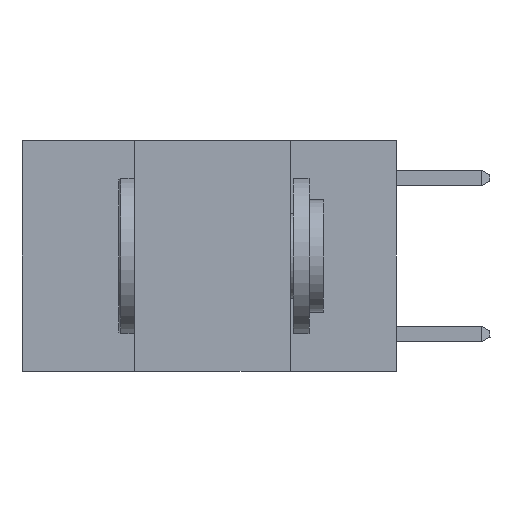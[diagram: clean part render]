
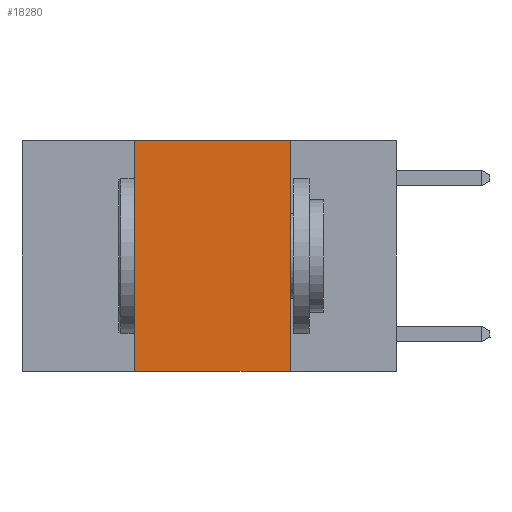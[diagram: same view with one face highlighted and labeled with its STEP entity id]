
A CAD part, left-side view. The second image highlights one B-rep face of the part: STEP entity #18280.
In plain terms, the highlighted planar face has unit normal (-1, 0, 0).
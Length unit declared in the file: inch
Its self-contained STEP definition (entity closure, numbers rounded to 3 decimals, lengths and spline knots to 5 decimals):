
#63 = VERTEX_POINT ( 'NONE', #12417 ) ;
#98 = CARTESIAN_POINT ( 'NONE',  ( 0., 0.42, -0.37 ) ) ;
#126 = CARTESIAN_POINT ( 'NONE',  ( 0., 0.6, 0. ) ) ;
#166 = LINE ( 'NONE', #17073, #260 ) ;
#260 = VECTOR ( 'NONE', #4436, 39.37008 ) ;
#839 = CARTESIAN_POINT ( 'NONE',  ( 0., 0.6, -0.37 ) ) ;
#1526 = EDGE_LOOP ( 'NONE', ( #18100, #18218, #18236, #18349 ) ) ;
#2316 = CARTESIAN_POINT ( 'NONE',  ( 0., 0.17, 0. ) ) ;
#2653 = CARTESIAN_POINT ( 'NONE',  ( 0., 0.42, 0. ) ) ;
#3962 = AXIS2_PLACEMENT_3D ( 'NONE', #126, #17803, #8577 ) ;
#4436 = DIRECTION ( 'NONE',  ( 0., -1., 0. ) ) ;
#5456 = VERTEX_POINT ( 'NONE', #18423 ) ;
#5472 = EDGE_CURVE ( 'NONE', #63, #5456, #166, .T. ) ;
#5507 = LINE ( 'NONE', #839, #5608 ) ;
#5608 = VECTOR ( 'NONE', #12369, 39.37008 ) ;
#6396 = VERTEX_POINT ( 'NONE', #9898 ) ;
#6684 = EDGE_CURVE ( 'NONE', #5456, #6396, #11560, .T. ) ;
#7364 = EDGE_CURVE ( 'NONE', #18940, #6396, #5507, .T. ) ;
#8577 = DIRECTION ( 'NONE',  ( 0., 0., -1. ) ) ;
#9541 = FACE_OUTER_BOUND ( 'NONE', #1526, .T. ) ;
#9898 = CARTESIAN_POINT ( 'NONE',  ( 0., 0.17, -0.37 ) ) ;
#10916 = VECTOR ( 'NONE', #14012, 39.37008 ) ;
#11374 = VECTOR ( 'NONE', #15243, 39.37008 ) ;
#11560 = LINE ( 'NONE', #2316, #11374 ) ;
#12369 = DIRECTION ( 'NONE',  ( 0., -1., 0. ) ) ;
#12408 = LINE ( 'NONE', #2653, #10916 ) ;
#12417 = CARTESIAN_POINT ( 'NONE',  ( 0., 0.42, 0. ) ) ;
#14012 = DIRECTION ( 'NONE',  ( 0., 0., 1. ) ) ;
#15243 = DIRECTION ( 'NONE',  ( 0., 0., -1. ) ) ;
#15854 = EDGE_CURVE ( 'NONE', #18940, #63, #12408, .T. ) ;
#16368 = PLANE ( 'NONE',  #3962 ) ;
#17073 = CARTESIAN_POINT ( 'NONE',  ( 0., 0.6, 0. ) ) ;
#17803 = DIRECTION ( 'NONE',  ( 1., 0., 0. ) ) ;
#18100 = ORIENTED_EDGE ( 'NONE', *, *, #6684, .F. ) ;
#18218 = ORIENTED_EDGE ( 'NONE', *, *, #5472, .F. ) ;
#18236 = ORIENTED_EDGE ( 'NONE', *, *, #15854, .F. ) ;
#18280 = ADVANCED_FACE ( 'NONE', ( #9541 ), #16368, .F. ) ;
#18349 = ORIENTED_EDGE ( 'NONE', *, *, #7364, .T. ) ;
#18423 = CARTESIAN_POINT ( 'NONE',  ( 0., 0.17, 0. ) ) ;
#18940 = VERTEX_POINT ( 'NONE', #98 ) ;
